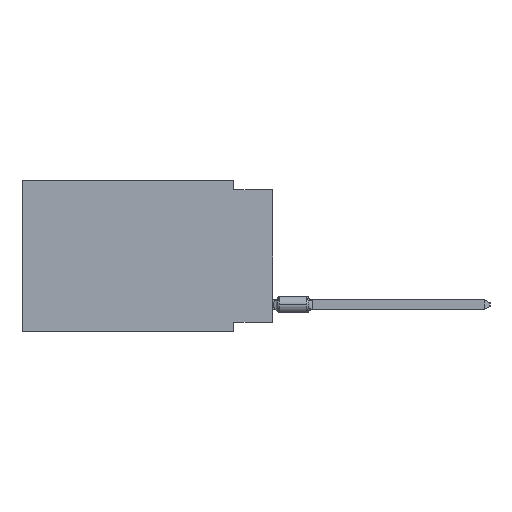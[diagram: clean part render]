
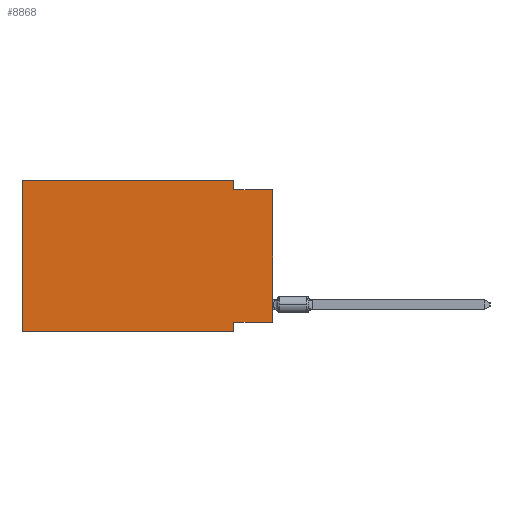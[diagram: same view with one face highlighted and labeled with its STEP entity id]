
A CAD part, left-side view. The second image highlights one B-rep face of the part: STEP entity #8868.
In plain terms, the highlighted planar face has unit normal (-1, 0, 0).
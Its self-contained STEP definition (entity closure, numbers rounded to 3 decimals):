
#2530 = CARTESIAN_POINT ( 'NONE',  ( 0., 2.54, 0. ) ) ;
#3135 = EDGE_LOOP ( 'NONE', ( #3963, #38016, #16425, #42357, #28260, #63063, #24957, #28047 ) ) ;
#3963 = ORIENTED_EDGE ( 'NONE', *, *, #45446, .T. ) ;
#6373 = CARTESIAN_POINT ( 'NONE',  ( 0., 0., -9.271 ) ) ;
#8304 = CARTESIAN_POINT ( 'NONE',  ( 0., 16.383, 0. ) ) ;
#8868 = ADVANCED_FACE ( 'NONE', ( #10603 ), #52019, .F. ) ;
#10603 = FACE_OUTER_BOUND ( 'NONE', #3135, .T. ) ;
#11492 = DIRECTION ( 'NONE',  ( 1., 0., 0. ) ) ;
#12775 = CARTESIAN_POINT ( 'NONE',  ( 0., 16.383, -9.906 ) ) ;
#13382 = VERTEX_POINT ( 'NONE', #64148 ) ;
#13978 = LINE ( 'NONE', #21092, #40474 ) ;
#14154 = VERTEX_POINT ( 'NONE', #84315 ) ;
#14210 = DIRECTION ( 'NONE',  ( 0., 0., -1. ) ) ;
#15170 = DIRECTION ( 'NONE',  ( 0., -1., 0. ) ) ;
#16425 = ORIENTED_EDGE ( 'NONE', *, *, #62291, .F. ) ;
#17388 = EDGE_CURVE ( 'NONE', #50640, #13382, #53301, .T. ) ;
#18070 = VECTOR ( 'NONE', #35215, 1000. ) ;
#20647 = DIRECTION ( 'NONE',  ( 0., 0., -1. ) ) ;
#21092 = CARTESIAN_POINT ( 'NONE',  ( 0., 2.54, -9.906 ) ) ;
#22221 = EDGE_CURVE ( 'NONE', #53655, #42018, #29384, .T. ) ;
#24957 = ORIENTED_EDGE ( 'NONE', *, *, #65441, .F. ) ;
#27981 = CARTESIAN_POINT ( 'NONE',  ( 0., 2.54, 0. ) ) ;
#28047 = ORIENTED_EDGE ( 'NONE', *, *, #83592, .F. ) ;
#28260 = ORIENTED_EDGE ( 'NONE', *, *, #68158, .F. ) ;
#29384 = LINE ( 'NONE', #56571, #45594 ) ;
#31069 = DIRECTION ( 'NONE',  ( 0., 0., -1. ) ) ;
#34225 = LINE ( 'NONE', #27981, #34591 ) ;
#34591 = VECTOR ( 'NONE', #14210, 1000. ) ;
#35215 = DIRECTION ( 'NONE',  ( 0., 0., 1. ) ) ;
#35444 = DIRECTION ( 'NONE',  ( 0., -1., 0. ) ) ;
#38016 = ORIENTED_EDGE ( 'NONE', *, *, #22221, .F. ) ;
#38198 = CARTESIAN_POINT ( 'NONE',  ( 0., 0., -9.271 ) ) ;
#40474 = VECTOR ( 'NONE', #20647, 1000. ) ;
#41432 = CARTESIAN_POINT ( 'NONE',  ( 0., 2.54, -0.635 ) ) ;
#42018 = VERTEX_POINT ( 'NONE', #82366 ) ;
#42357 = ORIENTED_EDGE ( 'NONE', *, *, #75545, .F. ) ;
#45446 = EDGE_CURVE ( 'NONE', #56168, #42018, #86980, .T. ) ;
#45594 = VECTOR ( 'NONE', #15170, 1000. ) ;
#50640 = VERTEX_POINT ( 'NONE', #51319 ) ;
#51319 = CARTESIAN_POINT ( 'NONE',  ( 0., 16.383, -9.906 ) ) ;
#52019 = PLANE ( 'NONE',  #85850 ) ;
#53120 = DIRECTION ( 'NONE',  ( 0., 0., 1. ) ) ;
#53301 = LINE ( 'NONE', #12775, #53938 ) ;
#53655 = VERTEX_POINT ( 'NONE', #41432 ) ;
#53938 = VECTOR ( 'NONE', #74232, 1000. ) ;
#55714 = CARTESIAN_POINT ( 'NONE',  ( 0., 16.383, 0. ) ) ;
#56168 = VERTEX_POINT ( 'NONE', #6373 ) ;
#56571 = CARTESIAN_POINT ( 'NONE',  ( 0., 0., -0.635 ) ) ;
#57515 = VERTEX_POINT ( 'NONE', #2530 ) ;
#58998 = VERTEX_POINT ( 'NONE', #66082 ) ;
#61529 = LINE ( 'NONE', #55714, #18070 ) ;
#62291 = EDGE_CURVE ( 'NONE', #57515, #53655, #34225, .T. ) ;
#63063 = ORIENTED_EDGE ( 'NONE', *, *, #17388, .T. ) ;
#64148 = CARTESIAN_POINT ( 'NONE',  ( 0., 2.54, -9.906 ) ) ;
#65441 = EDGE_CURVE ( 'NONE', #14154, #13382, #13978, .T. ) ;
#65840 = LINE ( 'NONE', #38198, #81847 ) ;
#66082 = CARTESIAN_POINT ( 'NONE',  ( 0., 16.383, 0. ) ) ;
#66269 = DIRECTION ( 'NONE',  ( 0., 1., 0. ) ) ;
#68158 = EDGE_CURVE ( 'NONE', #50640, #58998, #61529, .T. ) ;
#69314 = LINE ( 'NONE', #8304, #80954 ) ;
#72300 = CARTESIAN_POINT ( 'NONE',  ( 0., 0., 0. ) ) ;
#74232 = DIRECTION ( 'NONE',  ( 0., -1., 0. ) ) ;
#75545 = EDGE_CURVE ( 'NONE', #58998, #57515, #69314, .T. ) ;
#80954 = VECTOR ( 'NONE', #35444, 1000. ) ;
#81847 = VECTOR ( 'NONE', #66269, 1000. ) ;
#82366 = CARTESIAN_POINT ( 'NONE',  ( 0., 0., -0.635 ) ) ;
#83592 = EDGE_CURVE ( 'NONE', #56168, #14154, #65840, .T. ) ;
#84315 = CARTESIAN_POINT ( 'NONE',  ( 0., 2.54, -9.271 ) ) ;
#84891 = VECTOR ( 'NONE', #53120, 1000. ) ;
#85850 = AXIS2_PLACEMENT_3D ( 'NONE', #85878, #11492, #31069 ) ;
#85878 = CARTESIAN_POINT ( 'NONE',  ( 0., 16.383, 0. ) ) ;
#86980 = LINE ( 'NONE', #72300, #84891 ) ;
